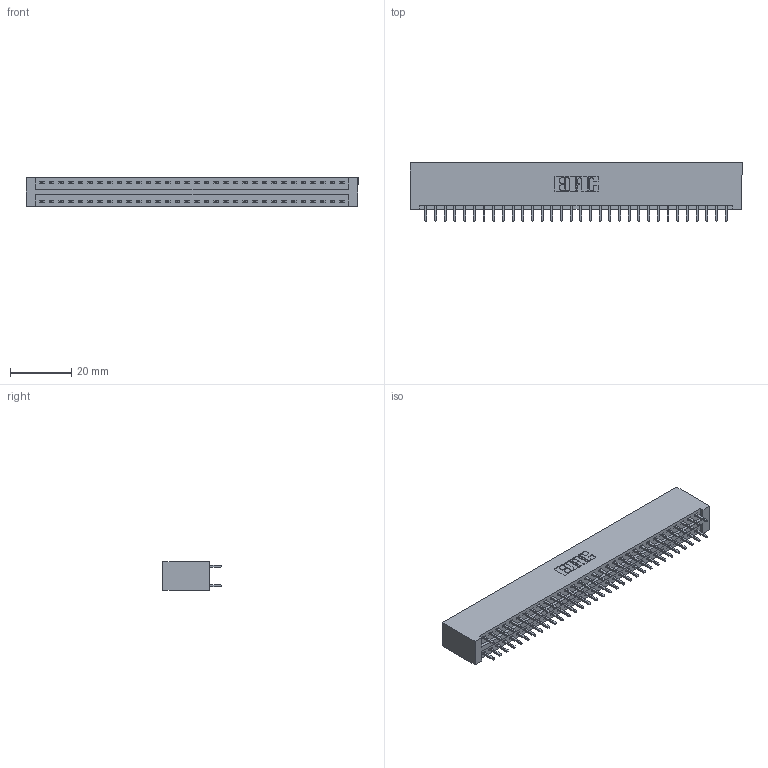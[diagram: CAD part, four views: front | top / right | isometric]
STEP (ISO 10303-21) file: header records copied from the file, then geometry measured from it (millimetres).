
FILE_DESCRIPTION (( 'STEP AP203' ), '1' );
FILE_NAME ('396-064-521-201.STEP', '2018-09-08T16:31:04', ( '' ), ( '' ), 'SwSTEP 2.0', 'SolidWorks 2016', '' );
FILE_SCHEMA (( 'CONFIG_CONTROL_DESIGN' ));
Length unit declared in the file: inch
Products named in the file (3): 396-064-521-201; 346 Part_No Mounting Lugs; 345-292-001_345-293-121
Assembly tree (65 placements, depth 2):
  396-064-521-201
    346 Part_No Mounting Lugs
    345-292-001_345-293-121  x64
Bounding box: 108.84 x 19.05 x 9.4 mm (x, y, z)
Volume: 11082.6 mm3; surface area: 15064 mm2
Topology: 65 solids, 65 shells, 3442 faces, 10225 edges, 6730 vertices
Faces by surface type: plane 2312, cylinder 1130
Entity records: 21971 total; most frequent: CARTESIAN_POINT 3632, ORIENTED_EDGE 3566, DIRECTION 3247, EDGE_CURVE 1783, LINE 1531, VECTOR 1531, VERTEX_POINT 1186, AXIS2_PLACEMENT_3D 858
